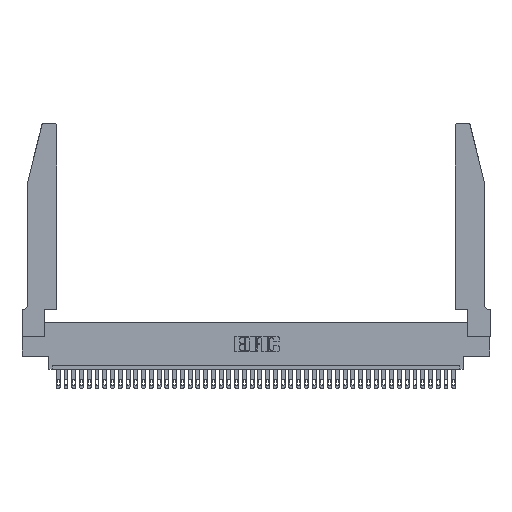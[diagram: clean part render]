
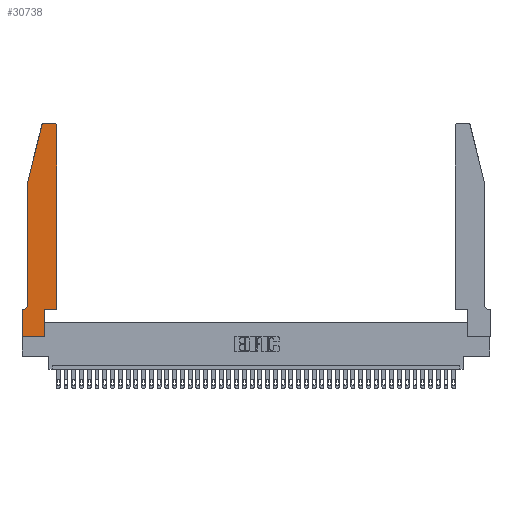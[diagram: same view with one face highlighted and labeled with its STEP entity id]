
A CAD part, top view. The second image highlights one B-rep face of the part: STEP entity #30738.
In plain terms, the highlighted planar face has unit normal (0, 0, 1).
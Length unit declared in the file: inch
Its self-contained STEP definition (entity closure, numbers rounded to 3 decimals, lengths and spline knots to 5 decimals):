
#232 = DIRECTION ( 'NONE',  ( 1., 0., 0. ) ) ;
#584 = DIRECTION ( 'NONE',  ( 1., 0., 0. ) ) ;
#993 = ORIENTED_EDGE ( 'NONE', *, *, #30898, .T. ) ;
#1456 = VERTEX_POINT ( 'NONE', #16826 ) ;
#1932 = CARTESIAN_POINT ( 'NONE',  ( 0., 0.35, 0.37 ) ) ;
#1944 = DIRECTION ( 'NONE',  ( -0.239, -0.971, 0. ) ) ;
#1987 = CARTESIAN_POINT ( 'NONE',  ( 0.0755, 2., 0.37 ) ) ;
#2037 = ORIENTED_EDGE ( 'NONE', *, *, #13943, .T. ) ;
#2086 = ORIENTED_EDGE ( 'NONE', *, *, #9229, .T. ) ;
#2325 = EDGE_CURVE ( 'NONE', #11349, #31604, #6896, .T. ) ;
#2425 = DIRECTION ( 'NONE',  ( 1., 0., 0. ) ) ;
#4613 = DIRECTION ( 'NONE',  ( 0., 1., 0. ) ) ;
#5152 = LINE ( 'NONE', #25430, #12816 ) ;
#5730 = CIRCLE ( 'NONE', #31529, 0.03 ) ;
#6570 = EDGE_CURVE ( 'NONE', #26839, #30367, #5152, .T. ) ;
#6674 = CARTESIAN_POINT ( 'NONE',  ( 0.4505, 0.35, 0.37 ) ) ;
#6854 = LINE ( 'NONE', #27389, #32081 ) ;
#6896 = LINE ( 'NONE', #19618, #7945 ) ;
#7065 = VERTEX_POINT ( 'NONE', #29477 ) ;
#7483 = DIRECTION ( 'NONE',  ( 1., 0., 0. ) ) ;
#7737 = ORIENTED_EDGE ( 'NONE', *, *, #41146, .T. ) ;
#7945 = VECTOR ( 'NONE', #232, 39.37008 ) ;
#7958 = EDGE_CURVE ( 'NONE', #30367, #38348, #21420, .T. ) ;
#9229 = EDGE_CURVE ( 'NONE', #22316, #20985, #22889, .T. ) ;
#9341 = VECTOR ( 'NONE', #13527, 39.37008 ) ;
#9549 = VERTEX_POINT ( 'NONE', #17473 ) ;
#9755 = ORIENTED_EDGE ( 'NONE', *, *, #2325, .T. ) ;
#10499 = VERTEX_POINT ( 'NONE', #15171 ) ;
#10538 = CARTESIAN_POINT ( 'NONE',  ( 0.2605, 2.75, 0.37 ) ) ;
#11349 = VERTEX_POINT ( 'NONE', #42368 ) ;
#11523 = FACE_OUTER_BOUND ( 'NONE', #20139, .T. ) ;
#11645 = DIRECTION ( 'NONE',  ( 0., -1., 0. ) ) ;
#11775 = EDGE_CURVE ( 'NONE', #38348, #7065, #36611, .T. ) ;
#12123 = EDGE_CURVE ( 'NONE', #9549, #10499, #5730, .T. ) ;
#12452 = AXIS2_PLACEMENT_3D ( 'NONE', #30816, #40766, #24184 ) ;
#12816 = VECTOR ( 'NONE', #28595, 39.37008 ) ;
#13527 = DIRECTION ( 'NONE',  ( -1., 0., 0. ) ) ;
#13943 = EDGE_CURVE ( 'NONE', #31604, #9549, #15543, .T. ) ;
#14283 = ORIENTED_EDGE ( 'NONE', *, *, #34243, .T. ) ;
#14661 = CARTESIAN_POINT ( 'NONE',  ( 0., 0., 0.37 ) ) ;
#14730 = CARTESIAN_POINT ( 'NONE',  ( 0.4505, 0.35, 0.37 ) ) ;
#15038 = ORIENTED_EDGE ( 'NONE', *, *, #7958, .T. ) ;
#15171 = CARTESIAN_POINT ( 'NONE',  ( 0.4205, 2.75, 0.37 ) ) ;
#15543 = LINE ( 'NONE', #6674, #36689 ) ;
#15641 = AXIS2_PLACEMENT_3D ( 'NONE', #40253, #40120, #7483 ) ;
#16826 = CARTESIAN_POINT ( 'NONE',  ( 0.284, 2.75, 0.37 ) ) ;
#16901 = DIRECTION ( 'NONE',  ( 0., 0., 1. ) ) ;
#17473 = CARTESIAN_POINT ( 'NONE',  ( 0.4505, 2.72, 0.37 ) ) ;
#18575 = VECTOR ( 'NONE', #584, 39.37008 ) ;
#19618 = CARTESIAN_POINT ( 'NONE',  ( 0.4505, 0.35, 0.37 ) ) ;
#19650 = CARTESIAN_POINT ( 'NONE',  ( 0., 0.35, 0.37 ) ) ;
#20139 = EDGE_LOOP ( 'NONE', ( #40086, #7737, #2086, #27620, #14283, #22053, #15038, #36349, #993, #9755, #2037, #39027 ) ) ;
#20985 = VERTEX_POINT ( 'NONE', #39194 ) ;
#21403 = EDGE_CURVE ( 'NONE', #20985, #36475, #25261, .T. ) ;
#21420 = LINE ( 'NONE', #14661, #27052 ) ;
#21780 = EDGE_CURVE ( 'NONE', #10499, #1456, #42286, .T. ) ;
#22053 = ORIENTED_EDGE ( 'NONE', *, *, #6570, .T. ) ;
#22316 = VERTEX_POINT ( 'NONE', #35694 ) ;
#22764 = CARTESIAN_POINT ( 'NONE',  ( 0.0755, 0.42, 0.37 ) ) ;
#22889 = LINE ( 'NONE', #27607, #30626 ) ;
#23595 = AXIS2_PLACEMENT_3D ( 'NONE', #19650, #16901, #40234 ) ;
#23709 = DIRECTION ( 'NONE',  ( 0., 1., 0. ) ) ;
#24184 = DIRECTION ( 'NONE',  ( -1., 0., 0. ) ) ;
#24214 = VECTOR ( 'NONE', #41646, 39.37008 ) ;
#25261 = LINE ( 'NONE', #1987, #24214 ) ;
#25430 = CARTESIAN_POINT ( 'NONE',  ( 0.0755, 0.35, 0.37 ) ) ;
#26839 = VERTEX_POINT ( 'NONE', #33989 ) ;
#27052 = VECTOR ( 'NONE', #11645, 39.37008 ) ;
#27389 = CARTESIAN_POINT ( 'NONE',  ( 0.2865, 0.35, 0.37 ) ) ;
#27607 = CARTESIAN_POINT ( 'NONE',  ( 0.0755, 2., 0.37 ) ) ;
#27620 = ORIENTED_EDGE ( 'NONE', *, *, #21403, .T. ) ;
#28500 = CARTESIAN_POINT ( 'NONE',  ( 0.4205, 2.72, 0.37 ) ) ;
#28595 = DIRECTION ( 'NONE',  ( -1., 0., 0. ) ) ;
#29477 = CARTESIAN_POINT ( 'NONE',  ( 0.2865, 0., 0.37 ) ) ;
#30367 = VERTEX_POINT ( 'NONE', #1932 ) ;
#30626 = VECTOR ( 'NONE', #1944, 39.37008 ) ;
#30738 = ADVANCED_FACE ( 'NONE', ( #11523 ), #36091, .T. ) ;
#30816 = CARTESIAN_POINT ( 'NONE',  ( 0.0055, 0.42, 0.37 ) ) ;
#30898 = EDGE_CURVE ( 'NONE', #7065, #11349, #6854, .T. ) ;
#31529 = AXIS2_PLACEMENT_3D ( 'NONE', #28500, #41785, #2425 ) ;
#31604 = VERTEX_POINT ( 'NONE', #14730 ) ;
#32081 = VECTOR ( 'NONE', #4613, 39.37008 ) ;
#32202 = CIRCLE ( 'NONE', #15641, 0.03 ) ;
#33989 = CARTESIAN_POINT ( 'NONE',  ( 0.0055, 0.35, 0.37 ) ) ;
#34243 = EDGE_CURVE ( 'NONE', #36475, #26839, #39885, .T. ) ;
#35694 = CARTESIAN_POINT ( 'NONE',  ( 0.25487, 2.72718, 0.37 ) ) ;
#35863 = CARTESIAN_POINT ( 'NONE',  ( 0., 0., 0.37 ) ) ;
#36091 = PLANE ( 'NONE',  #23595 ) ;
#36349 = ORIENTED_EDGE ( 'NONE', *, *, #11775, .T. ) ;
#36475 = VERTEX_POINT ( 'NONE', #22764 ) ;
#36611 = LINE ( 'NONE', #36677, #18575 ) ;
#36677 = CARTESIAN_POINT ( 'NONE',  ( 0., 0., 0.37 ) ) ;
#36689 = VECTOR ( 'NONE', #23709, 39.37008 ) ;
#38348 = VERTEX_POINT ( 'NONE', #35863 ) ;
#39027 = ORIENTED_EDGE ( 'NONE', *, *, #12123, .T. ) ;
#39194 = CARTESIAN_POINT ( 'NONE',  ( 0.0755, 2., 0.37 ) ) ;
#39885 = CIRCLE ( 'NONE', #12452, 0.07 ) ;
#40086 = ORIENTED_EDGE ( 'NONE', *, *, #21780, .T. ) ;
#40120 = DIRECTION ( 'NONE',  ( 0., 0., 1. ) ) ;
#40234 = DIRECTION ( 'NONE',  ( 1., 0., 0. ) ) ;
#40253 = CARTESIAN_POINT ( 'NONE',  ( 0.284, 2.72, 0.37 ) ) ;
#40766 = DIRECTION ( 'NONE',  ( 0., 0., -1. ) ) ;
#41146 = EDGE_CURVE ( 'NONE', #1456, #22316, #32202, .T. ) ;
#41646 = DIRECTION ( 'NONE',  ( 0., -1., 0. ) ) ;
#41785 = DIRECTION ( 'NONE',  ( 0., 0., 1. ) ) ;
#42286 = LINE ( 'NONE', #10538, #9341 ) ;
#42368 = CARTESIAN_POINT ( 'NONE',  ( 0.2865, 0.35, 0.37 ) ) ;
